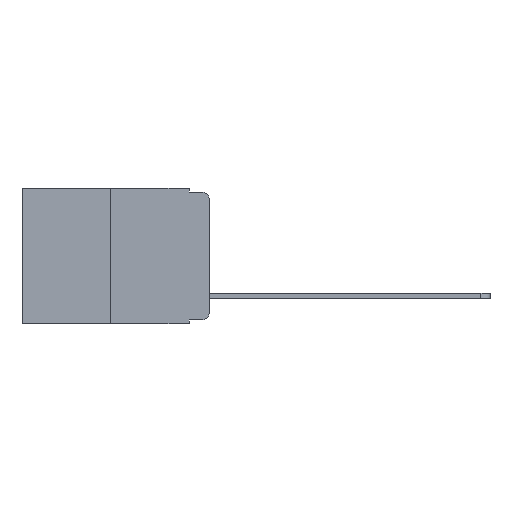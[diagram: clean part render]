
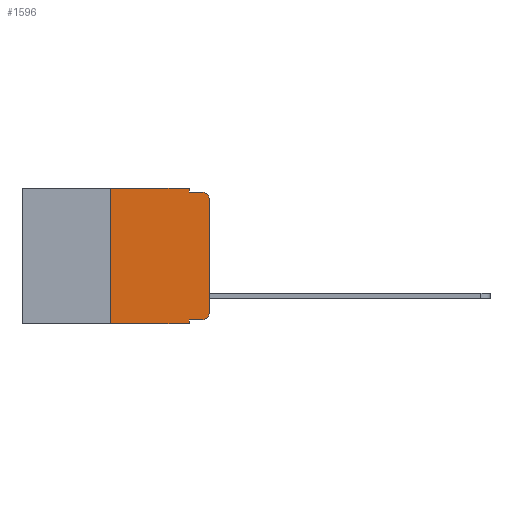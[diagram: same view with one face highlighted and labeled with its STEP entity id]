
A CAD part, left-side view. The second image highlights one B-rep face of the part: STEP entity #1596.
In plain terms, the highlighted planar face has unit normal (-1, 0, 0).
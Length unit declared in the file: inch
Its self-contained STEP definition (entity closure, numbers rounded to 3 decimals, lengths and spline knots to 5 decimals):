
#332 = VECTOR ( 'NONE', #9286, 39.37008 ) ;
#404 = EDGE_LOOP ( 'NONE', ( #7511, #11250, #9266, #1815, #1472, #9323, #11228, #5863, #5855, #6710 ) ) ;
#869 = VERTEX_POINT ( 'NONE', #8856 ) ;
#980 = LINE ( 'NONE', #3280, #332 ) ;
#1049 = CARTESIAN_POINT ( 'NONE',  ( 0., 0.02, -0.03 ) ) ;
#1138 = CARTESIAN_POINT ( 'NONE',  ( 0., 0., -0.03 ) ) ;
#1472 = ORIENTED_EDGE ( 'NONE', *, *, #10056, .F. ) ;
#1505 = VECTOR ( 'NONE', #10637, 39.37008 ) ;
#1596 = ADVANCED_FACE ( 'NONE', ( #9003 ), #1966, .F. ) ;
#1790 = DIRECTION ( 'NONE',  ( 0., -1., 0. ) ) ;
#1815 = ORIENTED_EDGE ( 'NONE', *, *, #11252, .F. ) ;
#1966 = PLANE ( 'NONE',  #3408 ) ;
#1967 = DIRECTION ( 'NONE',  ( 0., 0., -1. ) ) ;
#2269 = CARTESIAN_POINT ( 'NONE',  ( 0., 0.473, -0.343 ) ) ;
#2503 = VECTOR ( 'NONE', #6585, 39.37008 ) ;
#2622 = CARTESIAN_POINT ( 'NONE',  ( 0., 0.25, 0. ) ) ;
#2679 = VECTOR ( 'NONE', #10309, 39.37008 ) ;
#2776 = LINE ( 'NONE', #9921, #2503 ) ;
#3135 = CARTESIAN_POINT ( 'NONE',  ( 0., 0.473, 0. ) ) ;
#3280 = CARTESIAN_POINT ( 'NONE',  ( 0., 0.051, 0. ) ) ;
#3392 = CIRCLE ( 'NONE', #5095, 0.02 ) ;
#3408 = AXIS2_PLACEMENT_3D ( 'NONE', #10378, #5881, #10113 ) ;
#3599 = DIRECTION ( 'NONE',  ( -1., 0., 0. ) ) ;
#3607 = LINE ( 'NONE', #7711, #10124 ) ;
#3632 = VECTOR ( 'NONE', #8341, 39.37008 ) ;
#3722 = DIRECTION ( 'NONE',  ( 0., 0., -1. ) ) ;
#3908 = EDGE_CURVE ( 'NONE', #6715, #6911, #10015, .T. ) ;
#3925 = CARTESIAN_POINT ( 'NONE',  ( 0., 0.25, -0.343 ) ) ;
#4010 = VERTEX_POINT ( 'NONE', #10878 ) ;
#4062 = EDGE_CURVE ( 'NONE', #6911, #7760, #10634, .T. ) ;
#4438 = CARTESIAN_POINT ( 'NONE',  ( 0., 0.02, -0.313 ) ) ;
#4686 = VERTEX_POINT ( 'NONE', #9911 ) ;
#5041 = LINE ( 'NONE', #2622, #2679 ) ;
#5095 = AXIS2_PLACEMENT_3D ( 'NONE', #1049, #7239, #1967 ) ;
#5318 = CARTESIAN_POINT ( 'NONE',  ( 0., 0., -0.313 ) ) ;
#5466 = EDGE_CURVE ( 'NONE', #10034, #9451, #3607, .T. ) ;
#5629 = VECTOR ( 'NONE', #11049, 39.37008 ) ;
#5713 = VECTOR ( 'NONE', #9137, 39.37008 ) ;
#5715 = CARTESIAN_POINT ( 'NONE',  ( 0., 0.051, -0.01 ) ) ;
#5855 = ORIENTED_EDGE ( 'NONE', *, *, #6831, .T. ) ;
#5863 = ORIENTED_EDGE ( 'NONE', *, *, #7987, .F. ) ;
#5881 = DIRECTION ( 'NONE',  ( 1., 0., 0. ) ) ;
#6061 = CARTESIAN_POINT ( 'NONE',  ( 0., 0.051, -0.333 ) ) ;
#6585 = DIRECTION ( 'NONE',  ( 0., 0., -1. ) ) ;
#6710 = ORIENTED_EDGE ( 'NONE', *, *, #3908, .T. ) ;
#6715 = VERTEX_POINT ( 'NONE', #7626 ) ;
#6831 = EDGE_CURVE ( 'NONE', #4010, #6715, #7921, .T. ) ;
#6911 = VERTEX_POINT ( 'NONE', #5318 ) ;
#7239 = DIRECTION ( 'NONE',  ( -1., 0., 0. ) ) ;
#7511 = ORIENTED_EDGE ( 'NONE', *, *, #4062, .T. ) ;
#7626 = CARTESIAN_POINT ( 'NONE',  ( 0., 0.02, -0.333 ) ) ;
#7711 = CARTESIAN_POINT ( 'NONE',  ( 0., 0.051, -0.01 ) ) ;
#7760 = VERTEX_POINT ( 'NONE', #1138 ) ;
#7921 = LINE ( 'NONE', #6061, #5629 ) ;
#7987 = EDGE_CURVE ( 'NONE', #4010, #8796, #980, .T. ) ;
#8336 = EDGE_CURVE ( 'NONE', #7760, #9451, #3392, .T. ) ;
#8341 = DIRECTION ( 'NONE',  ( 0., -1., 0. ) ) ;
#8796 = VERTEX_POINT ( 'NONE', #10771 ) ;
#8800 = EDGE_CURVE ( 'NONE', #11207, #8796, #9666, .T. ) ;
#8856 = CARTESIAN_POINT ( 'NONE',  ( 0., 0.051, 0. ) ) ;
#9003 = FACE_OUTER_BOUND ( 'NONE', #404, .T. ) ;
#9061 = EDGE_CURVE ( 'NONE', #11207, #4686, #5041, .T. ) ;
#9137 = DIRECTION ( 'NONE',  ( 0., -1., 0. ) ) ;
#9162 = CARTESIAN_POINT ( 'NONE',  ( 0., 0.02, -0.01 ) ) ;
#9266 = ORIENTED_EDGE ( 'NONE', *, *, #5466, .F. ) ;
#9286 = DIRECTION ( 'NONE',  ( 0., 0., -1. ) ) ;
#9323 = ORIENTED_EDGE ( 'NONE', *, *, #9061, .F. ) ;
#9391 = AXIS2_PLACEMENT_3D ( 'NONE', #4438, #3599, #3722 ) ;
#9451 = VERTEX_POINT ( 'NONE', #9162 ) ;
#9666 = LINE ( 'NONE', #2269, #5713 ) ;
#9911 = CARTESIAN_POINT ( 'NONE',  ( 0., 0.25, 0. ) ) ;
#9921 = CARTESIAN_POINT ( 'NONE',  ( 0., 0.051, 0. ) ) ;
#10015 = CIRCLE ( 'NONE', #9391, 0.02 ) ;
#10034 = VERTEX_POINT ( 'NONE', #5715 ) ;
#10056 = EDGE_CURVE ( 'NONE', #4686, #869, #10403, .T. ) ;
#10113 = DIRECTION ( 'NONE',  ( 0., 0., -1. ) ) ;
#10124 = VECTOR ( 'NONE', #1790, 39.37008 ) ;
#10309 = DIRECTION ( 'NONE',  ( 0., 0., 1. ) ) ;
#10378 = CARTESIAN_POINT ( 'NONE',  ( 0., 0.473, 0. ) ) ;
#10403 = LINE ( 'NONE', #3135, #3632 ) ;
#10634 = LINE ( 'NONE', #10832, #1505 ) ;
#10637 = DIRECTION ( 'NONE',  ( 0., 0., 1. ) ) ;
#10771 = CARTESIAN_POINT ( 'NONE',  ( 0., 0.051, -0.343 ) ) ;
#10832 = CARTESIAN_POINT ( 'NONE',  ( 0., 0., 0. ) ) ;
#10878 = CARTESIAN_POINT ( 'NONE',  ( 0., 0.051, -0.333 ) ) ;
#11049 = DIRECTION ( 'NONE',  ( 0., -1., 0. ) ) ;
#11207 = VERTEX_POINT ( 'NONE', #3925 ) ;
#11228 = ORIENTED_EDGE ( 'NONE', *, *, #8800, .T. ) ;
#11250 = ORIENTED_EDGE ( 'NONE', *, *, #8336, .T. ) ;
#11252 = EDGE_CURVE ( 'NONE', #869, #10034, #2776, .T. ) ;
